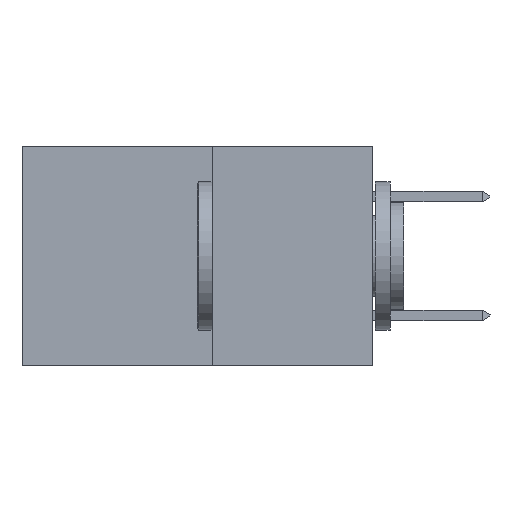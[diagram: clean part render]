
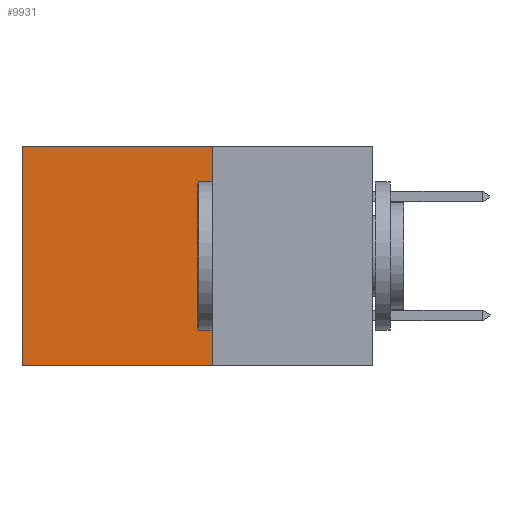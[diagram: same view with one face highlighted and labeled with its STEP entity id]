
A CAD part, left-side view. The second image highlights one B-rep face of the part: STEP entity #9931.
In plain terms, the highlighted planar face has unit normal (-1, 0, 0).
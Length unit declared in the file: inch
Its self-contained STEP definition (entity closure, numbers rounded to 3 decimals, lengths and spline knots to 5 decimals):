
#1181 = CARTESIAN_POINT ( 'NONE',  ( 0.277, 0.59, -0.37 ) ) ;
#2691 = LINE ( 'NONE', #8727, #21429 ) ;
#3703 = VERTEX_POINT ( 'NONE', #1181 ) ;
#3965 = CARTESIAN_POINT ( 'NONE',  ( 0.277, 0.27, 0. ) ) ;
#5148 = ORIENTED_EDGE ( 'NONE', *, *, #8121, .F. ) ;
#5478 = EDGE_CURVE ( 'NONE', #5501, #3703, #15195, .T. ) ;
#5501 = VERTEX_POINT ( 'NONE', #14013 ) ;
#6740 = EDGE_LOOP ( 'NONE', ( #14032, #5148, #20054, #7843 ) ) ;
#7843 = ORIENTED_EDGE ( 'NONE', *, *, #21574, .T. ) ;
#8121 = EDGE_CURVE ( 'NONE', #17736, #3703, #17081, .T. ) ;
#8727 = CARTESIAN_POINT ( 'NONE',  ( 0.277, 0.27, 0. ) ) ;
#9931 = ADVANCED_FACE ( 'NONE', ( #10589 ), #11725, .F. ) ;
#10589 = FACE_OUTER_BOUND ( 'NONE', #6740, .T. ) ;
#11379 = DIRECTION ( 'NONE',  ( 0., 0., -1. ) ) ;
#11464 = DIRECTION ( 'NONE',  ( 1., 0., 0. ) ) ;
#11672 = CARTESIAN_POINT ( 'NONE',  ( 0.277, 0.27, -0.37 ) ) ;
#11725 = PLANE ( 'NONE',  #14528 ) ;
#12389 = DIRECTION ( 'NONE',  ( 0., 1., 0. ) ) ;
#13162 = DIRECTION ( 'NONE',  ( 0., 0., -1. ) ) ;
#13720 = CARTESIAN_POINT ( 'NONE',  ( 0.277, 0.59, -0.37 ) ) ;
#14013 = CARTESIAN_POINT ( 'NONE',  ( 0.277, 0.59, 0. ) ) ;
#14032 = ORIENTED_EDGE ( 'NONE', *, *, #5478, .T. ) ;
#14103 = DIRECTION ( 'NONE',  ( 0., 1., 0. ) ) ;
#14109 = CARTESIAN_POINT ( 'NONE',  ( 0.277, 0.27, -0.37 ) ) ;
#14528 = AXIS2_PLACEMENT_3D ( 'NONE', #11672, #11464, #11379 ) ;
#15195 = LINE ( 'NONE', #13720, #19404 ) ;
#15906 = CARTESIAN_POINT ( 'NONE',  ( 0.277, 0.27, -0.37 ) ) ;
#16074 = VERTEX_POINT ( 'NONE', #3965 ) ;
#16965 = CARTESIAN_POINT ( 'NONE',  ( 0.277, 0.27, -0.37 ) ) ;
#17081 = LINE ( 'NONE', #14109, #22907 ) ;
#17595 = LINE ( 'NONE', #16965, #21725 ) ;
#17736 = VERTEX_POINT ( 'NONE', #15906 ) ;
#18822 = EDGE_CURVE ( 'NONE', #16074, #17736, #17595, .T. ) ;
#19404 = VECTOR ( 'NONE', #13162, 39.37008 ) ;
#20054 = ORIENTED_EDGE ( 'NONE', *, *, #18822, .F. ) ;
#20529 = DIRECTION ( 'NONE',  ( 0., 0., -1. ) ) ;
#21429 = VECTOR ( 'NONE', #12389, 39.37008 ) ;
#21574 = EDGE_CURVE ( 'NONE', #16074, #5501, #2691, .T. ) ;
#21725 = VECTOR ( 'NONE', #20529, 39.37008 ) ;
#22907 = VECTOR ( 'NONE', #14103, 39.37008 ) ;
